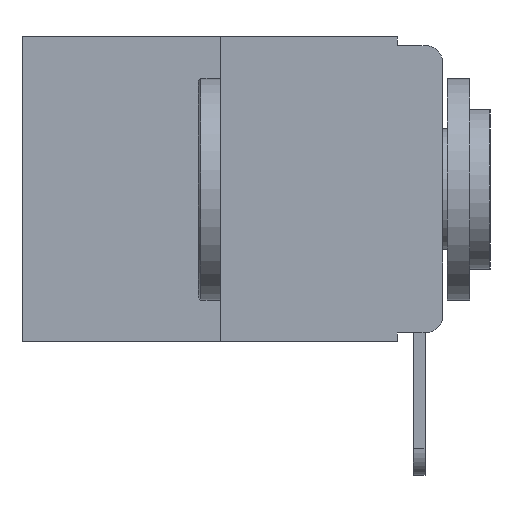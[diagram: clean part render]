
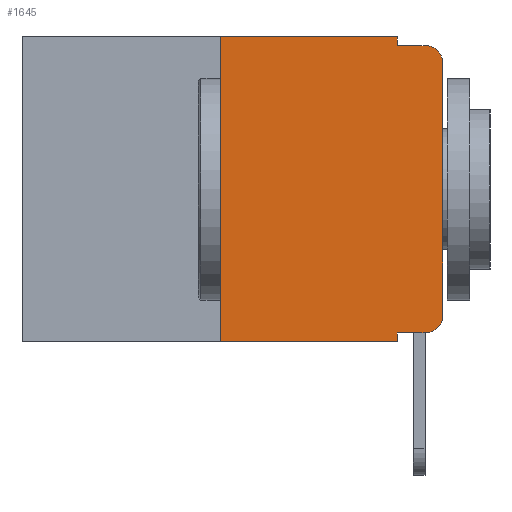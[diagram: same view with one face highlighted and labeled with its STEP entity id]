
A CAD part, left-side view. The second image highlights one B-rep face of the part: STEP entity #1645.
In plain terms, the highlighted planar face has unit normal (-1, 0, 0).
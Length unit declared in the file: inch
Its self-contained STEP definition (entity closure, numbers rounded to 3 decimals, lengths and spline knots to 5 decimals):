
#545 = CARTESIAN_POINT ( 'NONE',  ( 0., 0.051, -0.333 ) ) ;
#580 = CARTESIAN_POINT ( 'NONE',  ( 0., 0.02, -0.313 ) ) ;
#797 = CARTESIAN_POINT ( 'NONE',  ( 0., 0., -0.03 ) ) ;
#849 = LINE ( 'NONE', #10577, #10726 ) ;
#1049 = ORIENTED_EDGE ( 'NONE', *, *, #5220, .T. ) ;
#1285 = ORIENTED_EDGE ( 'NONE', *, *, #7486, .T. ) ;
#1540 = ORIENTED_EDGE ( 'NONE', *, *, #14610, .F. ) ;
#1645 = ADVANCED_FACE ( 'NONE', ( #10155 ), #7977, .F. ) ;
#1783 = DIRECTION ( 'NONE',  ( 0., 0., -1. ) ) ;
#1980 = EDGE_CURVE ( 'NONE', #6443, #12321, #10837, .T. ) ;
#2037 = DIRECTION ( 'NONE',  ( 0., 0., -1. ) ) ;
#2536 = ORIENTED_EDGE ( 'NONE', *, *, #6257, .T. ) ;
#2794 = DIRECTION ( 'NONE',  ( 0., 0., -1. ) ) ;
#2800 = EDGE_LOOP ( 'NONE', ( #1285, #1049, #9090, #1540, #5011, #6393, #7103, #5170, #3690, #2536 ) ) ;
#2810 = AXIS2_PLACEMENT_3D ( 'NONE', #9704, #5732, #1783 ) ;
#2874 = VECTOR ( 'NONE', #10990, 39.37008 ) ;
#2967 = DIRECTION ( 'NONE',  ( 0., 0., -1. ) ) ;
#3067 = CARTESIAN_POINT ( 'NONE',  ( 0., 0.473, 0. ) ) ;
#3401 = CARTESIAN_POINT ( 'NONE',  ( 0., 0.051, 0. ) ) ;
#3488 = VECTOR ( 'NONE', #5508, 39.37008 ) ;
#3496 = VERTEX_POINT ( 'NONE', #3401 ) ;
#3690 = ORIENTED_EDGE ( 'NONE', *, *, #10122, .T. ) ;
#4007 = VERTEX_POINT ( 'NONE', #6205 ) ;
#4078 = AXIS2_PLACEMENT_3D ( 'NONE', #580, #9042, #2037 ) ;
#4113 = CARTESIAN_POINT ( 'NONE',  ( 0., 0.02, -0.01 ) ) ;
#4253 = VERTEX_POINT ( 'NONE', #4795 ) ;
#4611 = CARTESIAN_POINT ( 'NONE',  ( 0., 0., -0.313 ) ) ;
#4692 = EDGE_CURVE ( 'NONE', #4007, #3496, #849, .T. ) ;
#4790 = CIRCLE ( 'NONE', #4078, 0.02 ) ;
#4795 = CARTESIAN_POINT ( 'NONE',  ( 0., 0.051, -0.343 ) ) ;
#4977 = AXIS2_PLACEMENT_3D ( 'NONE', #3067, #7099, #6383 ) ;
#5011 = ORIENTED_EDGE ( 'NONE', *, *, #4692, .F. ) ;
#5170 = ORIENTED_EDGE ( 'NONE', *, *, #11633, .F. ) ;
#5220 = EDGE_CURVE ( 'NONE', #9684, #12321, #10018, .T. ) ;
#5508 = DIRECTION ( 'NONE',  ( 0., 0., 1. ) ) ;
#5620 = DIRECTION ( 'NONE',  ( 0., 0., 1. ) ) ;
#5732 = DIRECTION ( 'NONE',  ( -1., 0., 0. ) ) ;
#6102 = LINE ( 'NONE', #9886, #9163 ) ;
#6205 = CARTESIAN_POINT ( 'NONE',  ( 0., 0.25, 0. ) ) ;
#6257 = EDGE_CURVE ( 'NONE', #8948, #11322, #4790, .T. ) ;
#6335 = LINE ( 'NONE', #9847, #2874 ) ;
#6383 = DIRECTION ( 'NONE',  ( 0., 0., -1. ) ) ;
#6393 = ORIENTED_EDGE ( 'NONE', *, *, #13113, .F. ) ;
#6443 = VERTEX_POINT ( 'NONE', #12700 ) ;
#6508 = LINE ( 'NONE', #7730, #3488 ) ;
#6609 = LINE ( 'NONE', #13557, #11585 ) ;
#6615 = DIRECTION ( 'NONE',  ( 0., -1., 0. ) ) ;
#7025 = CARTESIAN_POINT ( 'NONE',  ( 0., 0.473, -0.343 ) ) ;
#7099 = DIRECTION ( 'NONE',  ( 1., 0., 0. ) ) ;
#7103 = ORIENTED_EDGE ( 'NONE', *, *, #12023, .T. ) ;
#7156 = LINE ( 'NONE', #7025, #12858 ) ;
#7195 = VERTEX_POINT ( 'NONE', #10718 ) ;
#7252 = VECTOR ( 'NONE', #2794, 39.37008 ) ;
#7486 = EDGE_CURVE ( 'NONE', #11322, #9684, #6508, .T. ) ;
#7673 = CARTESIAN_POINT ( 'NONE',  ( 0., 0.051, -0.01 ) ) ;
#7730 = CARTESIAN_POINT ( 'NONE',  ( 0., 0., 0. ) ) ;
#7977 = PLANE ( 'NONE',  #4977 ) ;
#8851 = CARTESIAN_POINT ( 'NONE',  ( 0., 0.02, -0.333 ) ) ;
#8948 = VERTEX_POINT ( 'NONE', #8851 ) ;
#9042 = DIRECTION ( 'NONE',  ( -1., 0., 0. ) ) ;
#9090 = ORIENTED_EDGE ( 'NONE', *, *, #1980, .F. ) ;
#9163 = VECTOR ( 'NONE', #2967, 39.37008 ) ;
#9344 = DIRECTION ( 'NONE',  ( 0., -1., 0. ) ) ;
#9684 = VERTEX_POINT ( 'NONE', #797 ) ;
#9704 = CARTESIAN_POINT ( 'NONE',  ( 0., 0.02, -0.03 ) ) ;
#9847 = CARTESIAN_POINT ( 'NONE',  ( 0., 0.051, -0.333 ) ) ;
#9886 = CARTESIAN_POINT ( 'NONE',  ( 0., 0.051, 0. ) ) ;
#10018 = CIRCLE ( 'NONE', #2810, 0.02 ) ;
#10122 = EDGE_CURVE ( 'NONE', #13067, #8948, #6335, .T. ) ;
#10155 = FACE_OUTER_BOUND ( 'NONE', #2800, .T. ) ;
#10577 = CARTESIAN_POINT ( 'NONE',  ( 0., 0.473, 0. ) ) ;
#10718 = CARTESIAN_POINT ( 'NONE',  ( 0., 0.25, -0.343 ) ) ;
#10726 = VECTOR ( 'NONE', #9344, 39.37008 ) ;
#10837 = LINE ( 'NONE', #7673, #13812 ) ;
#10990 = DIRECTION ( 'NONE',  ( 0., -1., 0. ) ) ;
#11322 = VERTEX_POINT ( 'NONE', #4611 ) ;
#11585 = VECTOR ( 'NONE', #5620, 39.37008 ) ;
#11633 = EDGE_CURVE ( 'NONE', #13067, #4253, #6102, .T. ) ;
#12023 = EDGE_CURVE ( 'NONE', #7195, #4253, #7156, .T. ) ;
#12321 = VERTEX_POINT ( 'NONE', #4113 ) ;
#12700 = CARTESIAN_POINT ( 'NONE',  ( 0., 0.051, -0.01 ) ) ;
#12858 = VECTOR ( 'NONE', #14923, 39.37008 ) ;
#13067 = VERTEX_POINT ( 'NONE', #545 ) ;
#13113 = EDGE_CURVE ( 'NONE', #7195, #4007, #6609, .T. ) ;
#13557 = CARTESIAN_POINT ( 'NONE',  ( 0., 0.25, 0. ) ) ;
#13655 = LINE ( 'NONE', #14291, #7252 ) ;
#13812 = VECTOR ( 'NONE', #6615, 39.37008 ) ;
#14291 = CARTESIAN_POINT ( 'NONE',  ( 0., 0.051, 0. ) ) ;
#14610 = EDGE_CURVE ( 'NONE', #3496, #6443, #13655, .T. ) ;
#14923 = DIRECTION ( 'NONE',  ( 0., -1., 0. ) ) ;
